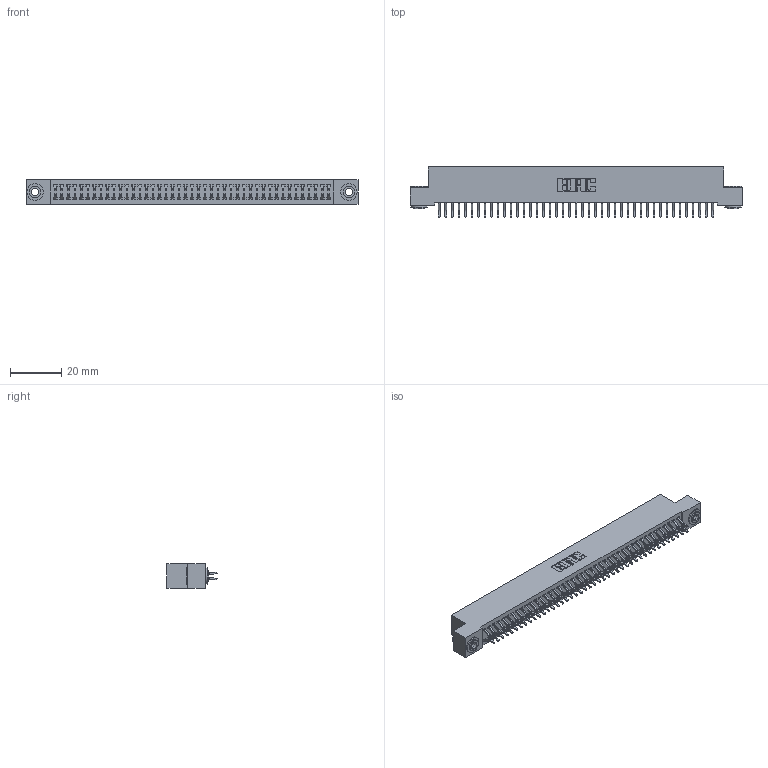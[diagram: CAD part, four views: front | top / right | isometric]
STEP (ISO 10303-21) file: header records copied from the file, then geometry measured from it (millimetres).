
FILE_DESCRIPTION (( 'STEP AP203' ), '1' );
FILE_NAME ('392-086-556-203.STEP', '2019-10-09T16:24:27', ( '' ), ( '' ), 'SwSTEP 2.0', 'SolidWorks 2016', '' );
FILE_SCHEMA (( 'CONFIG_CONTROL_DESIGN' ));
Length unit declared in the file: inch
Products named in the file (4): 392-086-556-203; 342 Part_.156 TH; 345-292-001_556 Tail; 342-250-002_345-250-002-102
Assembly tree (89 placements, depth 2):
  392-086-556-203
    342 Part_.156 TH
    345-292-001_556 Tail  x86
    342-250-002_345-250-002-102  x2
Bounding box: 129.54 x 19.58 x 9.4 mm (x, y, z)
Volume: 11664.5 mm3; surface area: 19142.2 mm2
Topology: 89 solids, 89 shells, 5136 faces, 15253 edges, 10050 vertices
Faces by surface type: plane 3516, cylinder 1612, cone 8
Entity records: 28272 total; most frequent: CARTESIAN_POINT 4673, ORIENTED_EDGE 4590, DIRECTION 4013, EDGE_CURVE 2295, VECTOR 2135, LINE 2135, VERTEX_POINT 1526, AXIS2_PLACEMENT_3D 939
